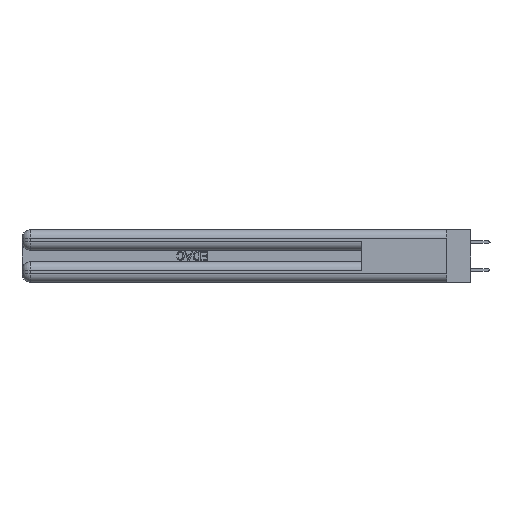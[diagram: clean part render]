
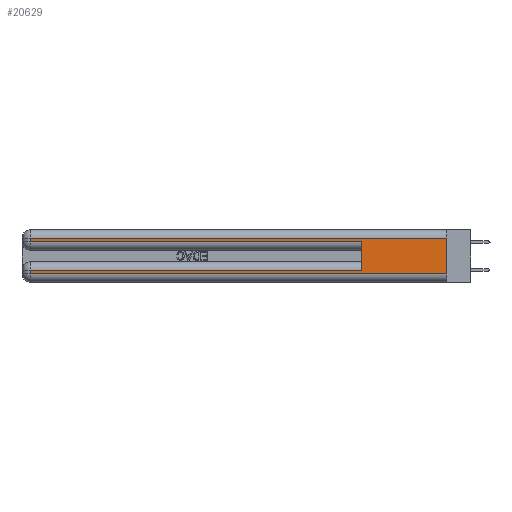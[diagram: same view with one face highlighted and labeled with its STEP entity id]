
A CAD part, left-side view. The second image highlights one B-rep face of the part: STEP entity #20629.
In plain terms, the highlighted planar face has unit normal (-1, 0, 0).
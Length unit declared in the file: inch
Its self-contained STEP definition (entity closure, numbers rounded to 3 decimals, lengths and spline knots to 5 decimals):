
#161 = EDGE_CURVE ( 'NONE', #30233, #6801, #6845, .T. ) ;
#2172 = LINE ( 'NONE', #14612, #3451 ) ;
#2283 = LINE ( 'NONE', #9143, #37001 ) ;
#3451 = VECTOR ( 'NONE', #23263, 39.37008 ) ;
#4010 = EDGE_CURVE ( 'NONE', #13982, #28004, #2283, .T. ) ;
#4141 = LINE ( 'NONE', #19008, #16385 ) ;
#4623 = CARTESIAN_POINT ( 'NONE',  ( 0., 2.94, 0.285 ) ) ;
#4911 = PLANE ( 'NONE',  #6436 ) ;
#4937 = LINE ( 'NONE', #5531, #29315 ) ;
#5085 = CARTESIAN_POINT ( 'NONE',  ( 0., 2.94, 0.31 ) ) ;
#5531 = CARTESIAN_POINT ( 'NONE',  ( 0., 0., 0.085 ) ) ;
#5805 = LINE ( 'NONE', #27283, #14996 ) ;
#5855 = VECTOR ( 'NONE', #12765, 39.37008 ) ;
#5989 = VERTEX_POINT ( 'NONE', #4623 ) ;
#6436 = AXIS2_PLACEMENT_3D ( 'NONE', #34846, #17148, #23000 ) ;
#6611 = LINE ( 'NONE', #31494, #33332 ) ;
#6801 = VERTEX_POINT ( 'NONE', #33017 ) ;
#6805 = ORIENTED_EDGE ( 'NONE', *, *, #35684, .F. ) ;
#6845 = LINE ( 'NONE', #28748, #32734 ) ;
#8149 = ORIENTED_EDGE ( 'NONE', *, *, #4010, .T. ) ;
#9143 = CARTESIAN_POINT ( 'NONE',  ( 0., 0., 0.31 ) ) ;
#9355 = CARTESIAN_POINT ( 'NONE',  ( 0., 0., 0.31 ) ) ;
#10713 = ORIENTED_EDGE ( 'NONE', *, *, #13799, .T. ) ;
#12102 = ORIENTED_EDGE ( 'NONE', *, *, #12403, .T. ) ;
#12403 = EDGE_CURVE ( 'NONE', #28004, #5989, #6611, .T. ) ;
#12608 = DIRECTION ( 'NONE',  ( 0., 0., -1. ) ) ;
#12765 = DIRECTION ( 'NONE',  ( 0., 0., -1. ) ) ;
#12826 = EDGE_LOOP ( 'NONE', ( #6805, #8149, #12102, #25780, #21679, #36941, #10713, #22806 ) ) ;
#13426 = VERTEX_POINT ( 'NONE', #21888 ) ;
#13799 = EDGE_CURVE ( 'NONE', #13426, #22089, #15765, .T. ) ;
#13982 = VERTEX_POINT ( 'NONE', #9355 ) ;
#14148 = FACE_OUTER_BOUND ( 'NONE', #12826, .T. ) ;
#14612 = CARTESIAN_POINT ( 'NONE',  ( 0., 0., 0.37 ) ) ;
#14996 = VECTOR ( 'NONE', #17632, 39.37008 ) ;
#15765 = LINE ( 'NONE', #28050, #5855 ) ;
#16057 = CARTESIAN_POINT ( 'NONE',  ( 0., 2.94, 0.06 ) ) ;
#16385 = VECTOR ( 'NONE', #25065, 39.37008 ) ;
#17148 = DIRECTION ( 'NONE',  ( 1., 0., 0. ) ) ;
#17632 = DIRECTION ( 'NONE',  ( 0., -1., 0. ) ) ;
#19008 = CARTESIAN_POINT ( 'NONE',  ( 0., 0., 0.06 ) ) ;
#20629 = ADVANCED_FACE ( 'NONE', ( #14148 ), #4911, .F. ) ;
#21679 = ORIENTED_EDGE ( 'NONE', *, *, #161, .F. ) ;
#21734 = DIRECTION ( 'NONE',  ( 0., 0., 1. ) ) ;
#21888 = CARTESIAN_POINT ( 'NONE',  ( 0., 2.94, 0.085 ) ) ;
#21950 = CARTESIAN_POINT ( 'NONE',  ( 0., 0., 0.06 ) ) ;
#22089 = VERTEX_POINT ( 'NONE', #16057 ) ;
#22806 = ORIENTED_EDGE ( 'NONE', *, *, #39464, .T. ) ;
#23000 = DIRECTION ( 'NONE',  ( 0., 0., -1. ) ) ;
#23263 = DIRECTION ( 'NONE',  ( 0., 0., -1. ) ) ;
#25065 = DIRECTION ( 'NONE',  ( 0., -1., 0. ) ) ;
#25780 = ORIENTED_EDGE ( 'NONE', *, *, #27205, .T. ) ;
#26807 = DIRECTION ( 'NONE',  ( 0., 1., 0. ) ) ;
#27205 = EDGE_CURVE ( 'NONE', #5989, #6801, #5805, .T. ) ;
#27283 = CARTESIAN_POINT ( 'NONE',  ( 0., 0., 0.285 ) ) ;
#28004 = VERTEX_POINT ( 'NONE', #5085 ) ;
#28050 = CARTESIAN_POINT ( 'NONE',  ( 0., 2.94, 0.37 ) ) ;
#28748 = CARTESIAN_POINT ( 'NONE',  ( 0., 0.6, 0.145 ) ) ;
#29315 = VECTOR ( 'NONE', #32639, 39.37008 ) ;
#30233 = VERTEX_POINT ( 'NONE', #38828 ) ;
#31494 = CARTESIAN_POINT ( 'NONE',  ( 0., 2.94, 0.37 ) ) ;
#32189 = VERTEX_POINT ( 'NONE', #21950 ) ;
#32639 = DIRECTION ( 'NONE',  ( 0., 1., 0. ) ) ;
#32734 = VECTOR ( 'NONE', #21734, 39.37008 ) ;
#32839 = EDGE_CURVE ( 'NONE', #30233, #13426, #4937, .T. ) ;
#33017 = CARTESIAN_POINT ( 'NONE',  ( 0., 0.6, 0.285 ) ) ;
#33332 = VECTOR ( 'NONE', #12608, 39.37008 ) ;
#34846 = CARTESIAN_POINT ( 'NONE',  ( 0., 0., 0.37 ) ) ;
#35684 = EDGE_CURVE ( 'NONE', #13982, #32189, #2172, .T. ) ;
#36941 = ORIENTED_EDGE ( 'NONE', *, *, #32839, .T. ) ;
#37001 = VECTOR ( 'NONE', #26807, 39.37008 ) ;
#38828 = CARTESIAN_POINT ( 'NONE',  ( 0., 0.6, 0.085 ) ) ;
#39464 = EDGE_CURVE ( 'NONE', #22089, #32189, #4141, .T. ) ;
